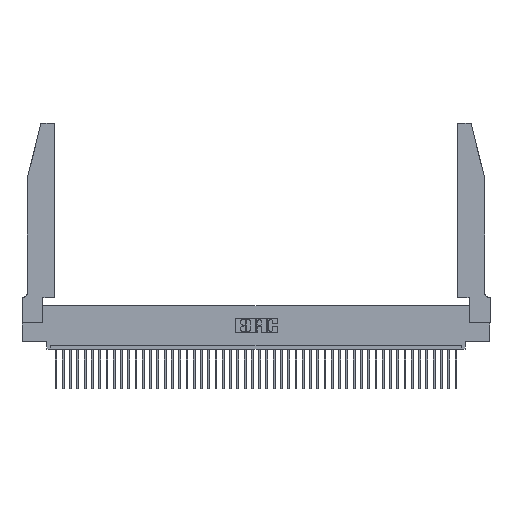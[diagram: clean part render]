
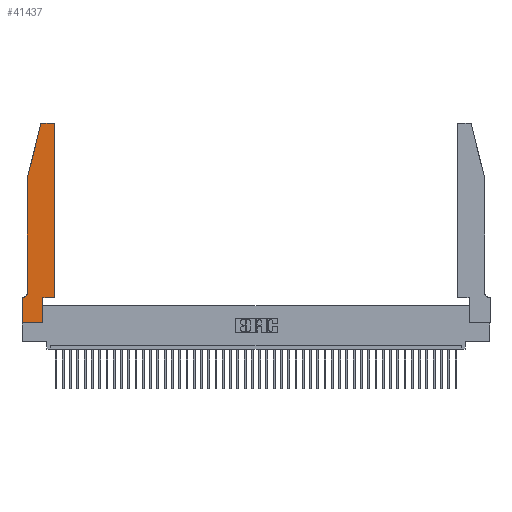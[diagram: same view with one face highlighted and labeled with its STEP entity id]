
A CAD part, top view. The second image highlights one B-rep face of the part: STEP entity #41437.
In plain terms, the highlighted planar face has unit normal (0, 0, 1).
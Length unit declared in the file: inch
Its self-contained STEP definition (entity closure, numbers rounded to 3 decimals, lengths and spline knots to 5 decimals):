
#508 = CARTESIAN_POINT ( 'NONE',  ( 0.0755, 0.42, 0.37 ) ) ;
#624 = CARTESIAN_POINT ( 'NONE',  ( 0.284, 2.75, 0.37 ) ) ;
#888 = LINE ( 'NONE', #18106, #43453 ) ;
#1455 = CARTESIAN_POINT ( 'NONE',  ( 0.2865, 0., 0.37 ) ) ;
#2274 = LINE ( 'NONE', #23736, #10474 ) ;
#2657 = EDGE_CURVE ( 'NONE', #8151, #37556, #19236, .T. ) ;
#3695 = ORIENTED_EDGE ( 'NONE', *, *, #11748, .T. ) ;
#3757 = EDGE_CURVE ( 'NONE', #42174, #8151, #3981, .T. ) ;
#3949 = CARTESIAN_POINT ( 'NONE',  ( 0.4505, 0.35, 0.37 ) ) ;
#3981 = LINE ( 'NONE', #22942, #30764 ) ;
#4571 = AXIS2_PLACEMENT_3D ( 'NONE', #13488, #29409, #40597 ) ;
#4747 = EDGE_CURVE ( 'NONE', #18549, #41654, #43667, .T. ) ;
#4903 = LINE ( 'NONE', #20359, #18597 ) ;
#5984 = DIRECTION ( 'NONE',  ( 0., -1., 0. ) ) ;
#7494 = CARTESIAN_POINT ( 'NONE',  ( 0.25487, 2.72718, 0.37 ) ) ;
#7822 = CARTESIAN_POINT ( 'NONE',  ( 0., 0.35, 0.37 ) ) ;
#8008 = ORIENTED_EDGE ( 'NONE', *, *, #37066, .T. ) ;
#8151 = VERTEX_POINT ( 'NONE', #27452 ) ;
#8349 = EDGE_CURVE ( 'NONE', #29481, #24795, #18887, .T. ) ;
#8817 = VERTEX_POINT ( 'NONE', #7494 ) ;
#9498 = CIRCLE ( 'NONE', #36815, 0.07 ) ;
#9570 = DIRECTION ( 'NONE',  ( 0., 0., 1. ) ) ;
#9620 = VECTOR ( 'NONE', #44003, 39.37008 ) ;
#10168 = ORIENTED_EDGE ( 'NONE', *, *, #3757, .T. ) ;
#10474 = VECTOR ( 'NONE', #37595, 39.37008 ) ;
#10775 = VERTEX_POINT ( 'NONE', #624 ) ;
#10970 = VECTOR ( 'NONE', #33590, 39.37008 ) ;
#11545 = VERTEX_POINT ( 'NONE', #33344 ) ;
#11748 = EDGE_CURVE ( 'NONE', #38496, #43258, #12032, .T. ) ;
#12032 = LINE ( 'NONE', #29734, #29508 ) ;
#13488 = CARTESIAN_POINT ( 'NONE',  ( 0., 0.35, 0.37 ) ) ;
#14553 = ORIENTED_EDGE ( 'NONE', *, *, #25308, .T. ) ;
#16207 = CARTESIAN_POINT ( 'NONE',  ( 0.0755, 0.35, 0.37 ) ) ;
#16501 = CARTESIAN_POINT ( 'NONE',  ( 0.2865, 0.35, 0.37 ) ) ;
#17649 = CARTESIAN_POINT ( 'NONE',  ( 0., 0., 0.37 ) ) ;
#18106 = CARTESIAN_POINT ( 'NONE',  ( 0.2605, 2.75, 0.37 ) ) ;
#18549 = VERTEX_POINT ( 'NONE', #25894 ) ;
#18597 = VECTOR ( 'NONE', #5984, 39.37008 ) ;
#18780 = ORIENTED_EDGE ( 'NONE', *, *, #28004, .T. ) ;
#18887 = LINE ( 'NONE', #33218, #9620 ) ;
#18968 = AXIS2_PLACEMENT_3D ( 'NONE', #36610, #36909, #23054 ) ;
#19236 = CIRCLE ( 'NONE', #37249, 0.03 ) ;
#19517 = ORIENTED_EDGE ( 'NONE', *, *, #4747, .T. ) ;
#19880 = EDGE_CURVE ( 'NONE', #24795, #11545, #20902, .T. ) ;
#20241 = CARTESIAN_POINT ( 'NONE',  ( 0.4205, 2.72, 0.37 ) ) ;
#20359 = CARTESIAN_POINT ( 'NONE',  ( 0., 0., 0.37 ) ) ;
#20475 = ORIENTED_EDGE ( 'NONE', *, *, #28173, .T. ) ;
#20902 = LINE ( 'NONE', #16501, #31294 ) ;
#22013 = CARTESIAN_POINT ( 'NONE',  ( 0.0055, 0.42, 0.37 ) ) ;
#22892 = ORIENTED_EDGE ( 'NONE', *, *, #8349, .T. ) ;
#22942 = CARTESIAN_POINT ( 'NONE',  ( 0.4505, 0.35, 0.37 ) ) ;
#23054 = DIRECTION ( 'NONE',  ( 1., 0., 0. ) ) ;
#23736 = CARTESIAN_POINT ( 'NONE',  ( 0.4505, 0.35, 0.37 ) ) ;
#23740 = DIRECTION ( 'NONE',  ( 1., 0., 0. ) ) ;
#24795 = VERTEX_POINT ( 'NONE', #1455 ) ;
#25308 = EDGE_CURVE ( 'NONE', #43258, #18549, #9498, .T. ) ;
#25591 = CARTESIAN_POINT ( 'NONE',  ( 0.4205, 2.75, 0.37 ) ) ;
#25894 = CARTESIAN_POINT ( 'NONE',  ( 0.0055, 0.35, 0.37 ) ) ;
#26887 = ORIENTED_EDGE ( 'NONE', *, *, #27432, .T. ) ;
#27322 = EDGE_LOOP ( 'NONE', ( #40651, #8008, #20475, #3695, #14553, #19517, #18780, #22892, #44231, #26887, #10168, #28224 ) ) ;
#27432 = EDGE_CURVE ( 'NONE', #11545, #42174, #2274, .T. ) ;
#27452 = CARTESIAN_POINT ( 'NONE',  ( 0.4505, 2.72, 0.37 ) ) ;
#28004 = EDGE_CURVE ( 'NONE', #41654, #29481, #4903, .T. ) ;
#28173 = EDGE_CURVE ( 'NONE', #8817, #38496, #29497, .T. ) ;
#28224 = ORIENTED_EDGE ( 'NONE', *, *, #2657, .T. ) ;
#28249 = CARTESIAN_POINT ( 'NONE',  ( 0.0755, 2., 0.37 ) ) ;
#28346 = VECTOR ( 'NONE', #41697, 39.37008 ) ;
#28727 = DIRECTION ( 'NONE',  ( -1., 0., 0. ) ) ;
#28930 = DIRECTION ( 'NONE',  ( -1., 0., 0. ) ) ;
#29409 = DIRECTION ( 'NONE',  ( 0., 0., 1. ) ) ;
#29481 = VERTEX_POINT ( 'NONE', #17649 ) ;
#29497 = LINE ( 'NONE', #28249, #28346 ) ;
#29508 = VECTOR ( 'NONE', #43263, 39.37008 ) ;
#29734 = CARTESIAN_POINT ( 'NONE',  ( 0.0755, 2., 0.37 ) ) ;
#30764 = VECTOR ( 'NONE', #39985, 39.37008 ) ;
#31148 = EDGE_CURVE ( 'NONE', #37556, #10775, #888, .T. ) ;
#31294 = VECTOR ( 'NONE', #40881, 39.37008 ) ;
#32401 = DIRECTION ( 'NONE',  ( 0., 0., -1. ) ) ;
#33218 = CARTESIAN_POINT ( 'NONE',  ( 0., 0., 0.37 ) ) ;
#33344 = CARTESIAN_POINT ( 'NONE',  ( 0.2865, 0.35, 0.37 ) ) ;
#33411 = FACE_OUTER_BOUND ( 'NONE', #27322, .T. ) ;
#33469 = PLANE ( 'NONE',  #4571 ) ;
#33590 = DIRECTION ( 'NONE',  ( -1., 0., 0. ) ) ;
#33919 = CARTESIAN_POINT ( 'NONE',  ( 0.0755, 2., 0.37 ) ) ;
#36610 = CARTESIAN_POINT ( 'NONE',  ( 0.284, 2.72, 0.37 ) ) ;
#36815 = AXIS2_PLACEMENT_3D ( 'NONE', #22013, #32401, #28727 ) ;
#36909 = DIRECTION ( 'NONE',  ( 0., 0., 1. ) ) ;
#37066 = EDGE_CURVE ( 'NONE', #10775, #8817, #38366, .T. ) ;
#37249 = AXIS2_PLACEMENT_3D ( 'NONE', #20241, #9570, #23740 ) ;
#37556 = VERTEX_POINT ( 'NONE', #25591 ) ;
#37595 = DIRECTION ( 'NONE',  ( 1., 0., 0. ) ) ;
#38366 = CIRCLE ( 'NONE', #18968, 0.03 ) ;
#38496 = VERTEX_POINT ( 'NONE', #33919 ) ;
#39985 = DIRECTION ( 'NONE',  ( 0., 1., 0. ) ) ;
#40597 = DIRECTION ( 'NONE',  ( 1., 0., 0. ) ) ;
#40651 = ORIENTED_EDGE ( 'NONE', *, *, #31148, .T. ) ;
#40881 = DIRECTION ( 'NONE',  ( 0., 1., 0. ) ) ;
#41437 = ADVANCED_FACE ( 'NONE', ( #33411 ), #33469, .T. ) ;
#41654 = VERTEX_POINT ( 'NONE', #7822 ) ;
#41697 = DIRECTION ( 'NONE',  ( -0.239, -0.971, 0. ) ) ;
#42174 = VERTEX_POINT ( 'NONE', #3949 ) ;
#43258 = VERTEX_POINT ( 'NONE', #508 ) ;
#43263 = DIRECTION ( 'NONE',  ( 0., -1., 0. ) ) ;
#43453 = VECTOR ( 'NONE', #28930, 39.37008 ) ;
#43667 = LINE ( 'NONE', #16207, #10970 ) ;
#44003 = DIRECTION ( 'NONE',  ( 1., 0., 0. ) ) ;
#44231 = ORIENTED_EDGE ( 'NONE', *, *, #19880, .T. ) ;
